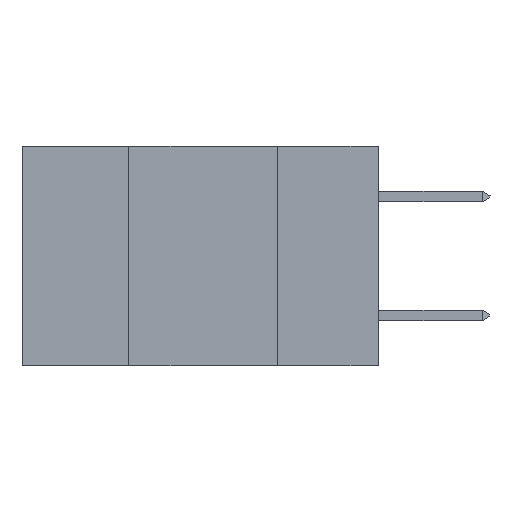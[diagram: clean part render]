
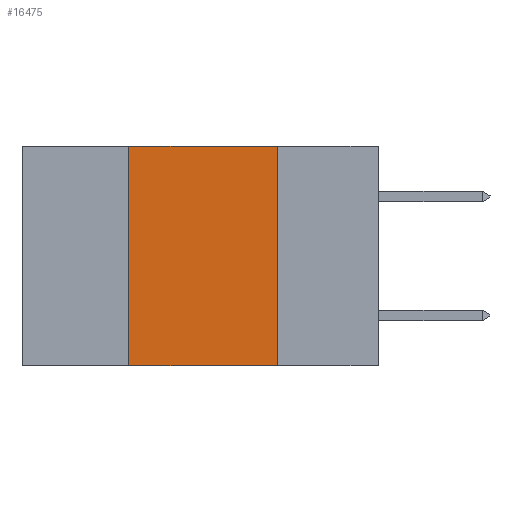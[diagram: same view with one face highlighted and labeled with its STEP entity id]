
A CAD part, left-side view. The second image highlights one B-rep face of the part: STEP entity #16475.
In plain terms, the highlighted planar face has unit normal (-1, 0, 0).
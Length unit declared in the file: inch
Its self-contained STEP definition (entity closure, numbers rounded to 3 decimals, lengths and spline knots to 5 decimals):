
#1218 = DIRECTION ( 'NONE',  ( 0., -1., 0. ) ) ;
#1479 = CARTESIAN_POINT ( 'NONE',  ( 0., 0.6, 0. ) ) ;
#2041 = VECTOR ( 'NONE', #1218, 39.37008 ) ;
#3394 = EDGE_CURVE ( 'NONE', #16805, #16159, #13582, .T. ) ;
#4153 = CARTESIAN_POINT ( 'NONE',  ( 0., 0.6, 0. ) ) ;
#4530 = DIRECTION ( 'NONE',  ( 1., 0., 0. ) ) ;
#5390 = DIRECTION ( 'NONE',  ( 0., 0., 1. ) ) ;
#5870 = ORIENTED_EDGE ( 'NONE', *, *, #3394, .T. ) ;
#6711 = CARTESIAN_POINT ( 'NONE',  ( 0., 0.42, 0. ) ) ;
#6773 = DIRECTION ( 'NONE',  ( 0., 0., -1. ) ) ;
#8137 = CARTESIAN_POINT ( 'NONE',  ( 0., 0.17, -0.37 ) ) ;
#8626 = EDGE_LOOP ( 'NONE', ( #16448, #15919, #8928, #5870 ) ) ;
#8928 = ORIENTED_EDGE ( 'NONE', *, *, #14108, .F. ) ;
#10093 = DIRECTION ( 'NONE',  ( 0., -1., 0. ) ) ;
#10184 = VERTEX_POINT ( 'NONE', #6711 ) ;
#10269 = PLANE ( 'NONE',  #16226 ) ;
#10770 = EDGE_CURVE ( 'NONE', #10184, #16933, #17388, .T. ) ;
#12128 = FACE_OUTER_BOUND ( 'NONE', #8626, .T. ) ;
#12312 = EDGE_CURVE ( 'NONE', #16933, #16159, #18737, .T. ) ;
#12563 = VECTOR ( 'NONE', #10093, 39.37008 ) ;
#12798 = LINE ( 'NONE', #18707, #13677 ) ;
#13361 = CARTESIAN_POINT ( 'NONE',  ( 0., 0.17, 0. ) ) ;
#13582 = LINE ( 'NONE', #16138, #2041 ) ;
#13677 = VECTOR ( 'NONE', #5390, 39.37008 ) ;
#13988 = CARTESIAN_POINT ( 'NONE',  ( 0., 0.17, -0.37 ) ) ;
#14108 = EDGE_CURVE ( 'NONE', #16805, #10184, #12798, .T. ) ;
#15086 = VECTOR ( 'NONE', #6773, 39.37008 ) ;
#15919 = ORIENTED_EDGE ( 'NONE', *, *, #10770, .F. ) ;
#16005 = CARTESIAN_POINT ( 'NONE',  ( 0., 0.42, -0.37 ) ) ;
#16138 = CARTESIAN_POINT ( 'NONE',  ( 0., 0.6, -0.37 ) ) ;
#16159 = VERTEX_POINT ( 'NONE', #8137 ) ;
#16216 = DIRECTION ( 'NONE',  ( 0., 0., -1. ) ) ;
#16226 = AXIS2_PLACEMENT_3D ( 'NONE', #1479, #4530, #16216 ) ;
#16448 = ORIENTED_EDGE ( 'NONE', *, *, #12312, .F. ) ;
#16475 = ADVANCED_FACE ( 'NONE', ( #12128 ), #10269, .F. ) ;
#16805 = VERTEX_POINT ( 'NONE', #16005 ) ;
#16933 = VERTEX_POINT ( 'NONE', #13361 ) ;
#17388 = LINE ( 'NONE', #4153, #12563 ) ;
#18707 = CARTESIAN_POINT ( 'NONE',  ( 0., 0.42, -0.37 ) ) ;
#18737 = LINE ( 'NONE', #13988, #15086 ) ;
